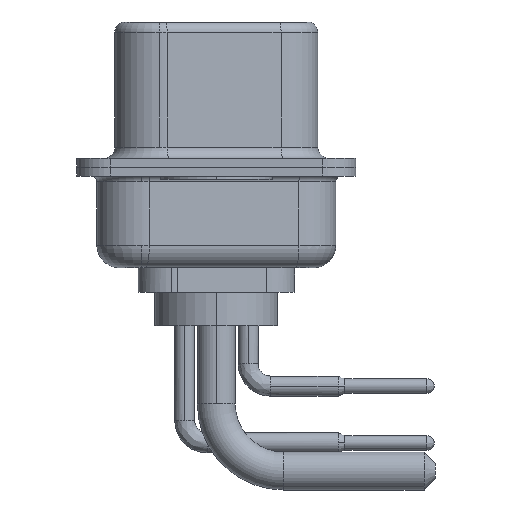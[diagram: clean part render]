
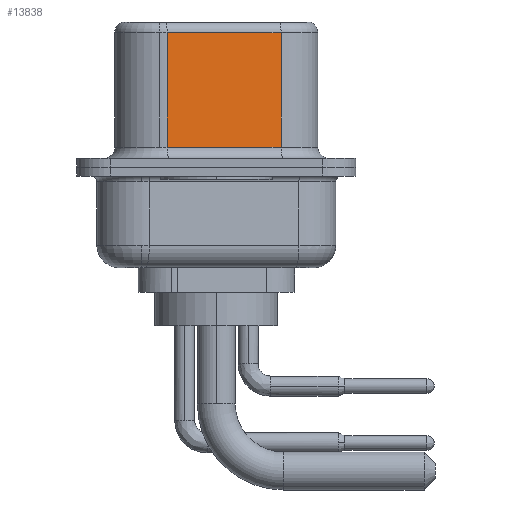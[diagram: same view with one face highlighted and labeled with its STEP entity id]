
A CAD part, left-side view. The second image highlights one B-rep face of the part: STEP entity #13838.
In plain terms, the highlighted planar face has unit normal (-0.985, -0.174, 0).
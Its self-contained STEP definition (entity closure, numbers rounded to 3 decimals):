
#751 = VECTOR ( 'NONE', #11442, 1000. ) ;
#789 = CARTESIAN_POINT ( 'NONE',  ( 4.555, -2.897, 6.52 ) ) ;
#951 = LINE ( 'NONE', #12744, #17652 ) ;
#1350 = EDGE_CURVE ( 'NONE', #12601, #8768, #17990, .T. ) ;
#2156 = DIRECTION ( 'NONE',  ( -0.174, 0.985, 0. ) ) ;
#2745 = ORIENTED_EDGE ( 'NONE', *, *, #1350, .T. ) ;
#3110 = CARTESIAN_POINT ( 'NONE',  ( 4.555, -2.897, 6.52 ) ) ;
#3188 = CARTESIAN_POINT ( 'NONE',  ( 4.555, -2.897, 0.9 ) ) ;
#3599 = VERTEX_POINT ( 'NONE', #7623 ) ;
#3801 = FACE_OUTER_BOUND ( 'NONE', #4071, .T. ) ;
#4071 = EDGE_LOOP ( 'NONE', ( #10059, #16446, #2745, #16916 ) ) ;
#4765 = LINE ( 'NONE', #3110, #7164 ) ;
#5372 = LINE ( 'NONE', #8637, #751 ) ;
#6410 = VERTEX_POINT ( 'NONE', #3188 ) ;
#6865 = DIRECTION ( 'NONE',  ( 0.174, -0.985, 0. ) ) ;
#7078 = EDGE_CURVE ( 'NONE', #3599, #12601, #5372, .T. ) ;
#7164 = VECTOR ( 'NONE', #17987, 1000. ) ;
#7623 = CARTESIAN_POINT ( 'NONE',  ( 4.555, -2.897, 6.02 ) ) ;
#8637 = CARTESIAN_POINT ( 'NONE',  ( 4.555, -2.897, 6.02 ) ) ;
#8768 = VERTEX_POINT ( 'NONE', #18672 ) ;
#9200 = DIRECTION ( 'NONE',  ( 0., 0., -1. ) ) ;
#9682 = PLANE ( 'NONE',  #14891 ) ;
#10059 = ORIENTED_EDGE ( 'NONE', *, *, #16687, .F. ) ;
#10698 = VECTOR ( 'NONE', #9200, 1000. ) ;
#11205 = CARTESIAN_POINT ( 'NONE',  ( 3.655, 2.203, 6.02 ) ) ;
#11442 = DIRECTION ( 'NONE',  ( -0.174, 0.985, 0. ) ) ;
#12601 = VERTEX_POINT ( 'NONE', #11205 ) ;
#12744 = CARTESIAN_POINT ( 'NONE',  ( 4.555, -2.897, 0.9 ) ) ;
#13838 = ADVANCED_FACE ( 'NONE', ( #3801 ), #9682, .F. ) ;
#14891 = AXIS2_PLACEMENT_3D ( 'NONE', #789, #15462, #2156 ) ;
#15462 = DIRECTION ( 'NONE',  ( 0.985, 0.174, 0. ) ) ;
#16446 = ORIENTED_EDGE ( 'NONE', *, *, #7078, .T. ) ;
#16687 = EDGE_CURVE ( 'NONE', #3599, #6410, #4765, .T. ) ;
#16852 = EDGE_CURVE ( 'NONE', #8768, #6410, #951, .T. ) ;
#16916 = ORIENTED_EDGE ( 'NONE', *, *, #16852, .T. ) ;
#17652 = VECTOR ( 'NONE', #6865, 1000. ) ;
#17987 = DIRECTION ( 'NONE',  ( 0., 0., -1. ) ) ;
#17990 = LINE ( 'NONE', #18089, #10698 ) ;
#18089 = CARTESIAN_POINT ( 'NONE',  ( 3.655, 2.203, 6.52 ) ) ;
#18672 = CARTESIAN_POINT ( 'NONE',  ( 3.655, 2.203, 0.9 ) ) ;
